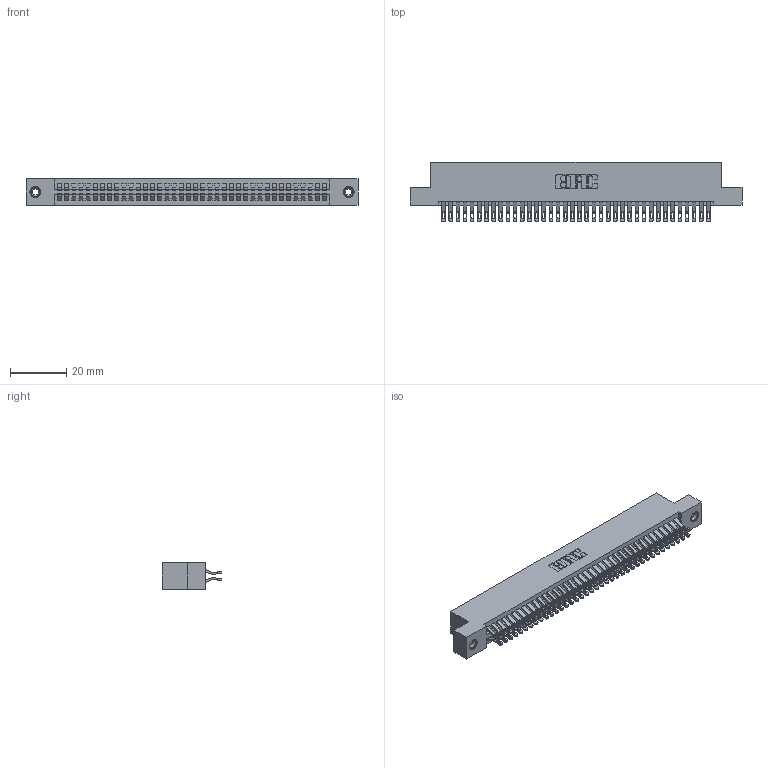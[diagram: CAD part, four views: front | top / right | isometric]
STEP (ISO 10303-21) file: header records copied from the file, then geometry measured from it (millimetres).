
FILE_DESCRIPTION (( 'STEP AP203' ), '1' );
FILE_NAME ('395-076-555-208.STEP', '2019-10-24T17:13:06', ( '' ), ( '' ), 'SwSTEP 2.0', 'SolidWorks 2016', '' );
FILE_SCHEMA (( 'CONFIG_CONTROL_DESIGN' ));
Length unit declared in the file: inch
Products named in the file (4): 395-076-555-208; 345 Part_Flush Mounting Lugs - 0.156 Dia-TI; 345-292-001_555 Tail; 345-250-001_345-250-003-102
Assembly tree (79 placements, depth 2):
  395-076-555-208
    345 Part_Flush Mounting Lugs - 0.156 Dia-TI
    345-292-001_555 Tail  x76
    345-250-001_345-250-003-102  x2
Bounding box: 117.73 x 21.13 x 9.4 mm (x, y, z)
Volume: 11613.1 mm3; surface area: 17868.8 mm2
Topology: 79 solids, 79 shells, 4442 faces, 13929 edges, 9278 vertices
Faces by surface type: plane 2468, cylinder 1958, cone 12, torus 4
Entity records: 31866 total; most frequent: CARTESIAN_POINT 5361, ORIENTED_EDGE 5258, DIRECTION 4727, EDGE_CURVE 2629, VECTOR 2305, LINE 2305, VERTEX_POINT 1748, AXIS2_PLACEMENT_3D 1211
